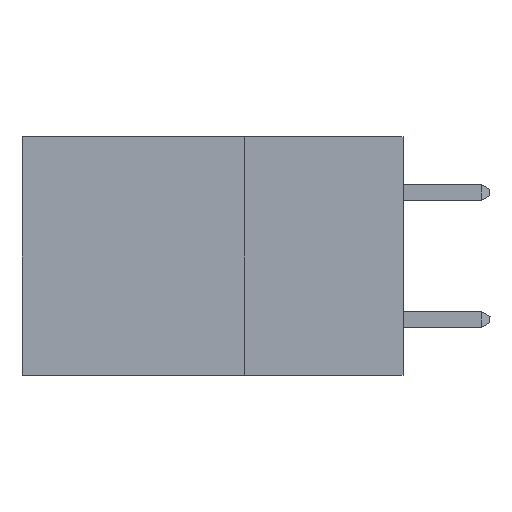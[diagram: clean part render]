
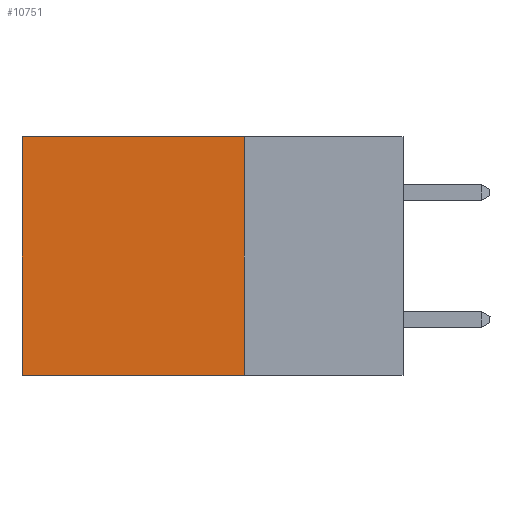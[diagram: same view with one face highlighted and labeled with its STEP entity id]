
A CAD part, left-side view. The second image highlights one B-rep face of the part: STEP entity #10751.
In plain terms, the highlighted planar face has unit normal (-1, 0, 0).
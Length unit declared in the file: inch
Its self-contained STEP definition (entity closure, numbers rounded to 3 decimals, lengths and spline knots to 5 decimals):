
#519 = CARTESIAN_POINT ( 'NONE',  ( 0.2875, 0.6, -0.375 ) ) ;
#584 = VERTEX_POINT ( 'NONE', #908 ) ;
#908 = CARTESIAN_POINT ( 'NONE',  ( 0.2875, 0.6, -0.375 ) ) ;
#1046 = CARTESIAN_POINT ( 'NONE',  ( 0.2875, 0.6, 0. ) ) ;
#1312 = VECTOR ( 'NONE', #7359, 39.37008 ) ;
#1539 = EDGE_CURVE ( 'NONE', #5559, #584, #9344, .T. ) ;
#1846 = CARTESIAN_POINT ( 'NONE',  ( 0.2875, 0.25, -0.375 ) ) ;
#2593 = CARTESIAN_POINT ( 'NONE',  ( 0.2875, 0.25, -0.375 ) ) ;
#3591 = CARTESIAN_POINT ( 'NONE',  ( 0.2875, 0.25, 0. ) ) ;
#3673 = LINE ( 'NONE', #519, #1312 ) ;
#3736 = CARTESIAN_POINT ( 'NONE',  ( 0.2875, 0.25, -0.375 ) ) ;
#4455 = VECTOR ( 'NONE', #13918, 39.37008 ) ;
#5559 = VERTEX_POINT ( 'NONE', #3736 ) ;
#5938 = VERTEX_POINT ( 'NONE', #13284 ) ;
#6115 = AXIS2_PLACEMENT_3D ( 'NONE', #21111, #12660, #14623 ) ;
#6143 = VECTOR ( 'NONE', #21320, 39.37008 ) ;
#7279 = ORIENTED_EDGE ( 'NONE', *, *, #20684, .T. ) ;
#7359 = DIRECTION ( 'NONE',  ( 0., 0., -1. ) ) ;
#7749 = EDGE_CURVE ( 'NONE', #5938, #17203, #12943, .T. ) ;
#7966 = LINE ( 'NONE', #2593, #6143 ) ;
#8811 = VECTOR ( 'NONE', #21371, 39.37008 ) ;
#9344 = LINE ( 'NONE', #1846, #8811 ) ;
#10639 = EDGE_LOOP ( 'NONE', ( #7279, #20743, #11418, #11040 ) ) ;
#10751 = ADVANCED_FACE ( 'NONE', ( #14723 ), #16133, .F. ) ;
#11040 = ORIENTED_EDGE ( 'NONE', *, *, #7749, .T. ) ;
#11418 = ORIENTED_EDGE ( 'NONE', *, *, #18128, .F. ) ;
#12660 = DIRECTION ( 'NONE',  ( 1., 0., 0. ) ) ;
#12943 = LINE ( 'NONE', #3591, #4455 ) ;
#13284 = CARTESIAN_POINT ( 'NONE',  ( 0.2875, 0.25, 0. ) ) ;
#13918 = DIRECTION ( 'NONE',  ( 0., 1., 0. ) ) ;
#14623 = DIRECTION ( 'NONE',  ( 0., 0., -1. ) ) ;
#14723 = FACE_OUTER_BOUND ( 'NONE', #10639, .T. ) ;
#16133 = PLANE ( 'NONE',  #6115 ) ;
#17203 = VERTEX_POINT ( 'NONE', #1046 ) ;
#18128 = EDGE_CURVE ( 'NONE', #5938, #5559, #7966, .T. ) ;
#20684 = EDGE_CURVE ( 'NONE', #17203, #584, #3673, .T. ) ;
#20743 = ORIENTED_EDGE ( 'NONE', *, *, #1539, .F. ) ;
#21111 = CARTESIAN_POINT ( 'NONE',  ( 0.2875, 0.25, -0.375 ) ) ;
#21320 = DIRECTION ( 'NONE',  ( 0., 0., -1. ) ) ;
#21371 = DIRECTION ( 'NONE',  ( 0., 1., 0. ) ) ;
